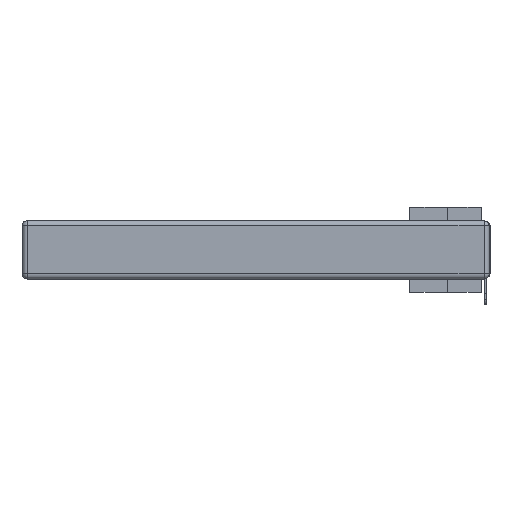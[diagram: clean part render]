
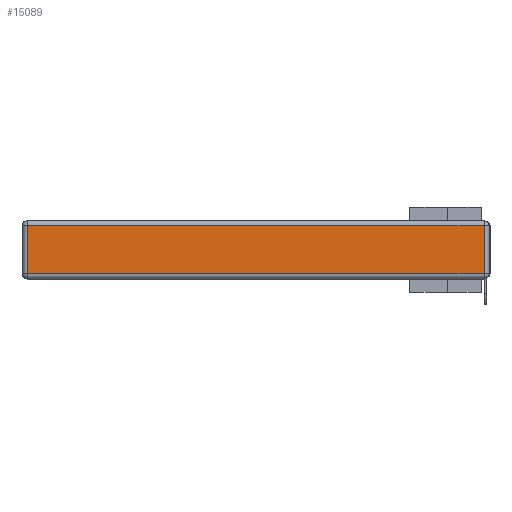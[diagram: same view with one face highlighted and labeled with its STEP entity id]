
A CAD part, left-side view. The second image highlights one B-rep face of the part: STEP entity #15089.
In plain terms, the highlighted planar face has unit normal (-1, 0, 0).
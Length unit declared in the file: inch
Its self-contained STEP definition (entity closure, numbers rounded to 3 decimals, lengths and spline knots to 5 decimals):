
#863 = CARTESIAN_POINT ( 'NONE',  ( 0., 0.03, -0.343 ) ) ;
#1283 = VECTOR ( 'NONE', #19971, 39.37008 ) ;
#1543 = VECTOR ( 'NONE', #19998, 39.37008 ) ;
#3486 = EDGE_CURVE ( 'NONE', #16530, #20299, #15628, .T. ) ;
#3620 = CARTESIAN_POINT ( 'NONE',  ( 0., 2.72, -0.313 ) ) ;
#3863 = DIRECTION ( 'NONE',  ( 0., 0., -1. ) ) ;
#4692 = CARTESIAN_POINT ( 'NONE',  ( 0., 0.03, -0.313 ) ) ;
#5483 = CARTESIAN_POINT ( 'NONE',  ( 0., 0., -0.313 ) ) ;
#10903 = CARTESIAN_POINT ( 'NONE',  ( 0., 2.72, -0.343 ) ) ;
#11143 = VECTOR ( 'NONE', #26536, 39.37008 ) ;
#11190 = EDGE_CURVE ( 'NONE', #29852, #26030, #17399, .T. ) ;
#12804 = CARTESIAN_POINT ( 'NONE',  ( 0., 0.03, -0.03 ) ) ;
#13473 = CARTESIAN_POINT ( 'NONE',  ( 0., 2.72, -0.03 ) ) ;
#13541 = ORIENTED_EDGE ( 'NONE', *, *, #27349, .T. ) ;
#15089 = ADVANCED_FACE ( 'NONE', ( #22018 ), #23861, .T. ) ;
#15278 = CARTESIAN_POINT ( 'NONE',  ( 0., 2.75, -0.03 ) ) ;
#15628 = LINE ( 'NONE', #10903, #22580 ) ;
#16530 = VERTEX_POINT ( 'NONE', #13473 ) ;
#17399 = LINE ( 'NONE', #863, #11143 ) ;
#17453 = EDGE_LOOP ( 'NONE', ( #13541, #25849, #17796, #27514 ) ) ;
#17796 = ORIENTED_EDGE ( 'NONE', *, *, #19908, .T. ) ;
#18164 = LINE ( 'NONE', #15278, #1543 ) ;
#19436 = DIRECTION ( 'NONE',  ( -1., 0., 0. ) ) ;
#19908 = EDGE_CURVE ( 'NONE', #26030, #16530, #18164, .T. ) ;
#19971 = DIRECTION ( 'NONE',  ( 0., -1., 0. ) ) ;
#19998 = DIRECTION ( 'NONE',  ( 0., 1., 0. ) ) ;
#20299 = VERTEX_POINT ( 'NONE', #3620 ) ;
#21670 = LINE ( 'NONE', #5483, #1283 ) ;
#21726 = CARTESIAN_POINT ( 'NONE',  ( 0., 0., -0.343 ) ) ;
#22018 = FACE_OUTER_BOUND ( 'NONE', #17453, .T. ) ;
#22580 = VECTOR ( 'NONE', #3863, 39.37008 ) ;
#23861 = PLANE ( 'NONE',  #29756 ) ;
#25849 = ORIENTED_EDGE ( 'NONE', *, *, #11190, .T. ) ;
#26030 = VERTEX_POINT ( 'NONE', #12804 ) ;
#26536 = DIRECTION ( 'NONE',  ( 0., 0., 1. ) ) ;
#27349 = EDGE_CURVE ( 'NONE', #20299, #29852, #21670, .T. ) ;
#27514 = ORIENTED_EDGE ( 'NONE', *, *, #3486, .T. ) ;
#29036 = DIRECTION ( 'NONE',  ( 0., 0., 1. ) ) ;
#29756 = AXIS2_PLACEMENT_3D ( 'NONE', #21726, #19436, #29036 ) ;
#29852 = VERTEX_POINT ( 'NONE', #4692 ) ;
